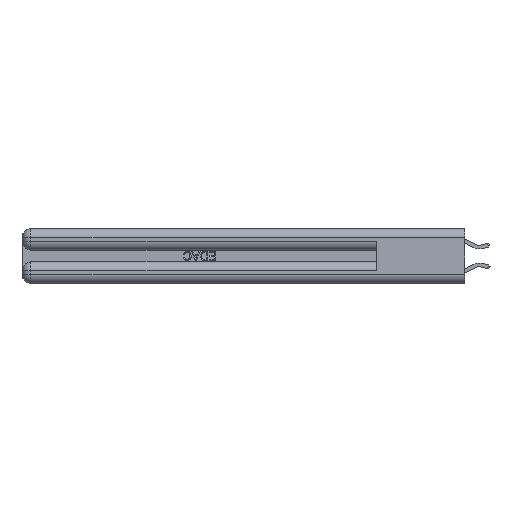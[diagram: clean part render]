
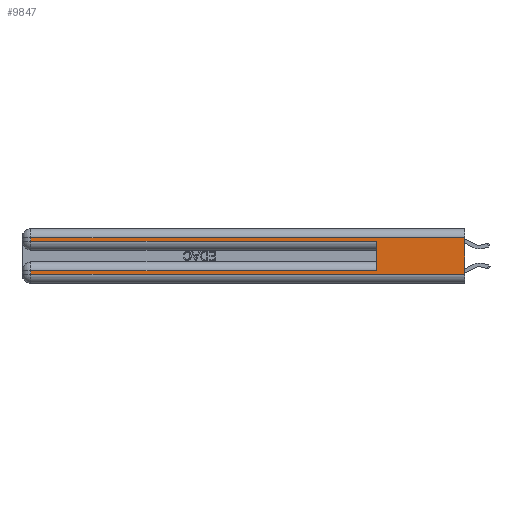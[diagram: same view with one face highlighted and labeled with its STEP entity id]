
A CAD part, left-side view. The second image highlights one B-rep face of the part: STEP entity #9847.
In plain terms, the highlighted planar face has unit normal (-1, 0, 0).
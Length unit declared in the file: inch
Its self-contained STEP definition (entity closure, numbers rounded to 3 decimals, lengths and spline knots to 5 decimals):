
#62 = VERTEX_POINT ( 'NONE', #6457 ) ;
#232 = VECTOR ( 'NONE', #27994, 39.37008 ) ;
#294 = LINE ( 'NONE', #27719, #26963 ) ;
#645 = EDGE_CURVE ( 'NONE', #25263, #5898, #20863, .T. ) ;
#689 = VERTEX_POINT ( 'NONE', #26093 ) ;
#1079 = VECTOR ( 'NONE', #31564, 39.37008 ) ;
#1241 = EDGE_CURVE ( 'NONE', #22086, #14957, #11208, .T. ) ;
#1604 = ORIENTED_EDGE ( 'NONE', *, *, #24625, .T. ) ;
#2384 = CARTESIAN_POINT ( 'NONE',  ( 0., 2.94, 0.37 ) ) ;
#3673 = FACE_OUTER_BOUND ( 'NONE', #23066, .T. ) ;
#4619 = CARTESIAN_POINT ( 'NONE',  ( 0., 0., 0.31 ) ) ;
#5757 = VERTEX_POINT ( 'NONE', #24224 ) ;
#5823 = DIRECTION ( 'NONE',  ( 0., 1., 0. ) ) ;
#5898 = VERTEX_POINT ( 'NONE', #6260 ) ;
#5909 = CARTESIAN_POINT ( 'NONE',  ( 0., 0.6, 0.085 ) ) ;
#6139 = CARTESIAN_POINT ( 'NONE',  ( 0., 0., 0.085 ) ) ;
#6260 = CARTESIAN_POINT ( 'NONE',  ( 0., 2.94, 0.31 ) ) ;
#6293 = PLANE ( 'NONE',  #10779 ) ;
#6457 = CARTESIAN_POINT ( 'NONE',  ( 0., 0.6, 0.285 ) ) ;
#8945 = VERTEX_POINT ( 'NONE', #5909 ) ;
#9241 = VECTOR ( 'NONE', #16158, 39.37008 ) ;
#9369 = VECTOR ( 'NONE', #13358, 39.37008 ) ;
#9847 = ADVANCED_FACE ( 'NONE', ( #3673 ), #6293, .F. ) ;
#10549 = CARTESIAN_POINT ( 'NONE',  ( 0., 0., 0.37 ) ) ;
#10561 = EDGE_CURVE ( 'NONE', #689, #62, #18775, .T. ) ;
#10779 = AXIS2_PLACEMENT_3D ( 'NONE', #26197, #21122, #31063 ) ;
#11056 = ORIENTED_EDGE ( 'NONE', *, *, #645, .T. ) ;
#11208 = LINE ( 'NONE', #31081, #1079 ) ;
#11250 = CARTESIAN_POINT ( 'NONE',  ( 0., 0., 0.31 ) ) ;
#12347 = LINE ( 'NONE', #2384, #24314 ) ;
#13358 = DIRECTION ( 'NONE',  ( 0., 1., 0. ) ) ;
#14336 = ORIENTED_EDGE ( 'NONE', *, *, #19657, .F. ) ;
#14957 = VERTEX_POINT ( 'NONE', #30662 ) ;
#15280 = CARTESIAN_POINT ( 'NONE',  ( 0., 2.94, 0.06 ) ) ;
#15425 = LINE ( 'NONE', #10549, #20962 ) ;
#16158 = DIRECTION ( 'NONE',  ( 0., -1., 0. ) ) ;
#16709 = ORIENTED_EDGE ( 'NONE', *, *, #32131, .T. ) ;
#18298 = CARTESIAN_POINT ( 'NONE',  ( 0., 0., 0.285 ) ) ;
#18504 = VECTOR ( 'NONE', #5823, 39.37008 ) ;
#18534 = LINE ( 'NONE', #6139, #18504 ) ;
#18775 = LINE ( 'NONE', #18298, #9241 ) ;
#19657 = EDGE_CURVE ( 'NONE', #25263, #14957, #15425, .T. ) ;
#20001 = LINE ( 'NONE', #29943, #232 ) ;
#20210 = ORIENTED_EDGE ( 'NONE', *, *, #31102, .T. ) ;
#20377 = DIRECTION ( 'NONE',  ( 0., 0., -1. ) ) ;
#20477 = DIRECTION ( 'NONE',  ( 0., 0., -1. ) ) ;
#20863 = LINE ( 'NONE', #11250, #9369 ) ;
#20962 = VECTOR ( 'NONE', #20477, 39.37008 ) ;
#21122 = DIRECTION ( 'NONE',  ( 1., 0., 0. ) ) ;
#22086 = VERTEX_POINT ( 'NONE', #15280 ) ;
#22098 = EDGE_CURVE ( 'NONE', #8945, #62, #20001, .T. ) ;
#22304 = DIRECTION ( 'NONE',  ( 0., 0., -1. ) ) ;
#23066 = EDGE_LOOP ( 'NONE', ( #14336, #11056, #16709, #26074, #28873, #1604, #20210, #31189 ) ) ;
#24224 = CARTESIAN_POINT ( 'NONE',  ( 0., 2.94, 0.085 ) ) ;
#24314 = VECTOR ( 'NONE', #22304, 39.37008 ) ;
#24625 = EDGE_CURVE ( 'NONE', #8945, #5757, #18534, .T. ) ;
#25263 = VERTEX_POINT ( 'NONE', #4619 ) ;
#26074 = ORIENTED_EDGE ( 'NONE', *, *, #10561, .T. ) ;
#26093 = CARTESIAN_POINT ( 'NONE',  ( 0., 2.94, 0.285 ) ) ;
#26197 = CARTESIAN_POINT ( 'NONE',  ( 0., 0., 0.37 ) ) ;
#26963 = VECTOR ( 'NONE', #20377, 39.37008 ) ;
#27719 = CARTESIAN_POINT ( 'NONE',  ( 0., 2.94, 0.37 ) ) ;
#27994 = DIRECTION ( 'NONE',  ( 0., 0., 1. ) ) ;
#28873 = ORIENTED_EDGE ( 'NONE', *, *, #22098, .F. ) ;
#29943 = CARTESIAN_POINT ( 'NONE',  ( 0., 0.6, 0.145 ) ) ;
#30662 = CARTESIAN_POINT ( 'NONE',  ( 0., 0., 0.06 ) ) ;
#31063 = DIRECTION ( 'NONE',  ( 0., 0., -1. ) ) ;
#31081 = CARTESIAN_POINT ( 'NONE',  ( 0., 0., 0.06 ) ) ;
#31102 = EDGE_CURVE ( 'NONE', #5757, #22086, #12347, .T. ) ;
#31189 = ORIENTED_EDGE ( 'NONE', *, *, #1241, .T. ) ;
#31564 = DIRECTION ( 'NONE',  ( 0., -1., 0. ) ) ;
#32131 = EDGE_CURVE ( 'NONE', #5898, #689, #294, .T. ) ;
